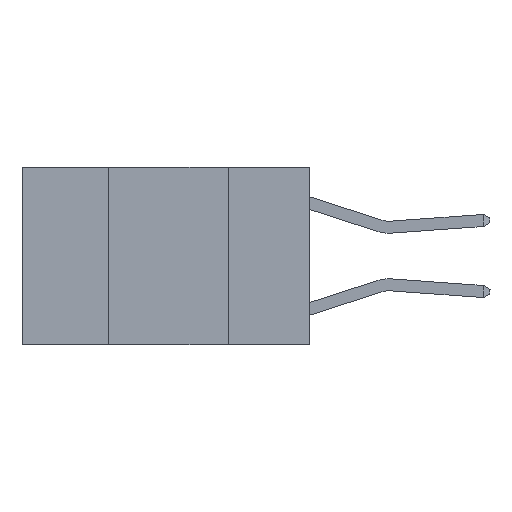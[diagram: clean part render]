
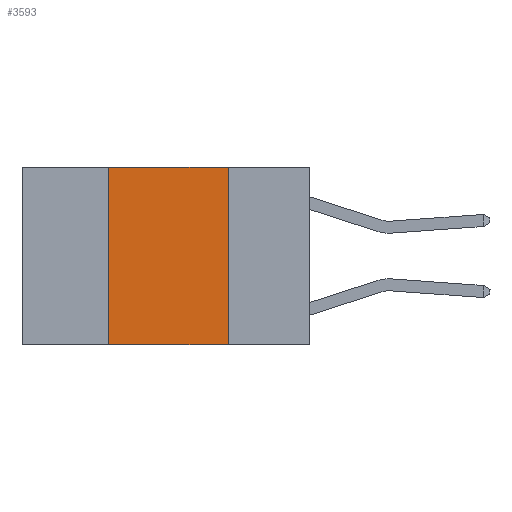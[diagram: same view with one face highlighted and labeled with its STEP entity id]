
A CAD part, left-side view. The second image highlights one B-rep face of the part: STEP entity #3593.
In plain terms, the highlighted planar face has unit normal (-1, 0, 0).
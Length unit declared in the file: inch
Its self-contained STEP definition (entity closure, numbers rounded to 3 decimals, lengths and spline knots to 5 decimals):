
#737 = AXIS2_PLACEMENT_3D ( 'NONE', #6199, #14961, #10606 ) ;
#836 = ORIENTED_EDGE ( 'NONE', *, *, #15751, .F. ) ;
#1270 = VERTEX_POINT ( 'NONE', #11037 ) ;
#1920 = VERTEX_POINT ( 'NONE', #5597 ) ;
#2003 = VERTEX_POINT ( 'NONE', #8546 ) ;
#2428 = DIRECTION ( 'NONE',  ( 0., -1., 0. ) ) ;
#3298 = CARTESIAN_POINT ( 'NONE',  ( 0., 0.6, 0. ) ) ;
#3593 = ADVANCED_FACE ( 'NONE', ( #6461 ), #11732, .F. ) ;
#3782 = LINE ( 'NONE', #7830, #4333 ) ;
#3927 = EDGE_LOOP ( 'NONE', ( #836, #12507, #7510, #15372 ) ) ;
#4333 = VECTOR ( 'NONE', #10495, 39.37008 ) ;
#4660 = LINE ( 'NONE', #3298, #16364 ) ;
#5097 = CARTESIAN_POINT ( 'NONE',  ( 0., 0.6, -0.37 ) ) ;
#5597 = CARTESIAN_POINT ( 'NONE',  ( 0., 0.42, 0. ) ) ;
#6199 = CARTESIAN_POINT ( 'NONE',  ( 0., 0.6, 0. ) ) ;
#6461 = FACE_OUTER_BOUND ( 'NONE', #3927, .T. ) ;
#7510 = ORIENTED_EDGE ( 'NONE', *, *, #13230, .F. ) ;
#7624 = DIRECTION ( 'NONE',  ( 0., -1., 0. ) ) ;
#7830 = CARTESIAN_POINT ( 'NONE',  ( 0., 0.42, 0. ) ) ;
#8257 = VECTOR ( 'NONE', #10786, 39.37008 ) ;
#8546 = CARTESIAN_POINT ( 'NONE',  ( 0., 0.17, -0.37 ) ) ;
#8738 = EDGE_CURVE ( 'NONE', #15888, #2003, #10441, .T. ) ;
#10441 = LINE ( 'NONE', #5097, #13315 ) ;
#10495 = DIRECTION ( 'NONE',  ( 0., 0., 1. ) ) ;
#10606 = DIRECTION ( 'NONE',  ( 0., 0., -1. ) ) ;
#10786 = DIRECTION ( 'NONE',  ( 0., 0., -1. ) ) ;
#11037 = CARTESIAN_POINT ( 'NONE',  ( 0., 0.17, 0. ) ) ;
#11251 = CARTESIAN_POINT ( 'NONE',  ( 0., 0.42, -0.37 ) ) ;
#11403 = EDGE_CURVE ( 'NONE', #1920, #1270, #4660, .T. ) ;
#11732 = PLANE ( 'NONE',  #737 ) ;
#11990 = CARTESIAN_POINT ( 'NONE',  ( 0., 0.17, 0. ) ) ;
#12507 = ORIENTED_EDGE ( 'NONE', *, *, #11403, .F. ) ;
#13230 = EDGE_CURVE ( 'NONE', #15888, #1920, #3782, .T. ) ;
#13315 = VECTOR ( 'NONE', #2428, 39.37008 ) ;
#14961 = DIRECTION ( 'NONE',  ( 1., 0., 0. ) ) ;
#15372 = ORIENTED_EDGE ( 'NONE', *, *, #8738, .T. ) ;
#15751 = EDGE_CURVE ( 'NONE', #1270, #2003, #17730, .T. ) ;
#15888 = VERTEX_POINT ( 'NONE', #11251 ) ;
#16364 = VECTOR ( 'NONE', #7624, 39.37008 ) ;
#17730 = LINE ( 'NONE', #11990, #8257 ) ;
